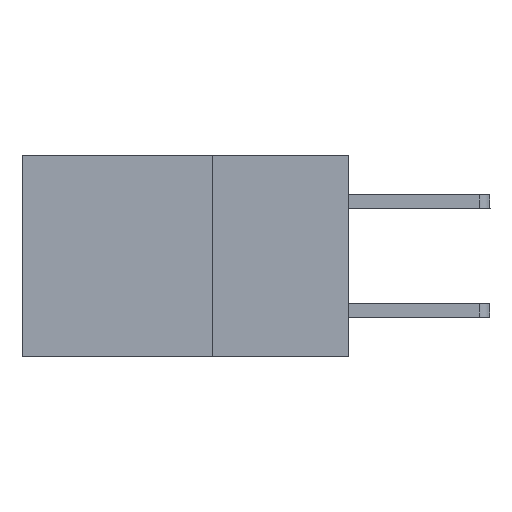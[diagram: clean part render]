
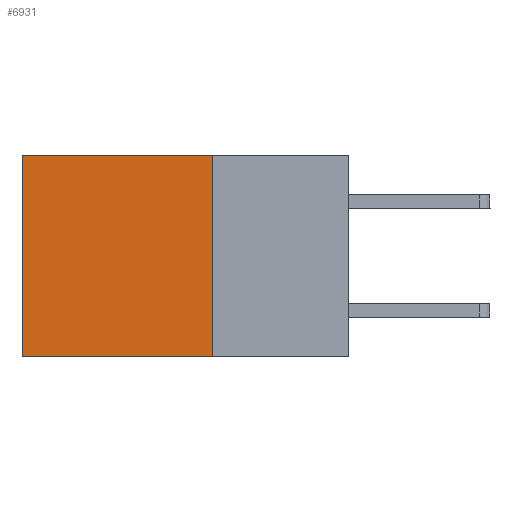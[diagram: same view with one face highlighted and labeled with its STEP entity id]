
A CAD part, left-side view. The second image highlights one B-rep face of the part: STEP entity #6931.
In plain terms, the highlighted planar face has unit normal (-1, 0, 0).
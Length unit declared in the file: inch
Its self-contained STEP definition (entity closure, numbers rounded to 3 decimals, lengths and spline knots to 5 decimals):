
#618 = VERTEX_POINT ( 'NONE', #10238 ) ;
#727 = CARTESIAN_POINT ( 'NONE',  ( 0.298, 0.25, -0.37 ) ) ;
#946 = CARTESIAN_POINT ( 'NONE',  ( 0.298, 0.6, 0. ) ) ;
#1016 = LINE ( 'NONE', #1638, #9282 ) ;
#1069 = ORIENTED_EDGE ( 'NONE', *, *, #3397, .F. ) ;
#1202 = VECTOR ( 'NONE', #9985, 39.37008 ) ;
#1638 = CARTESIAN_POINT ( 'NONE',  ( 0.298, 0.25, 0. ) ) ;
#2792 = DIRECTION ( 'NONE',  ( 0., 0., -1. ) ) ;
#2838 = DIRECTION ( 'NONE',  ( 1., 0., 0. ) ) ;
#3087 = AXIS2_PLACEMENT_3D ( 'NONE', #9989, #2838, #2792 ) ;
#3397 = EDGE_CURVE ( 'NONE', #8082, #6408, #9560, .T. ) ;
#3431 = DIRECTION ( 'NONE',  ( 0., 0., -1. ) ) ;
#3647 = CARTESIAN_POINT ( 'NONE',  ( 0.298, 0.25, 0. ) ) ;
#4001 = ORIENTED_EDGE ( 'NONE', *, *, #9084, .F. ) ;
#4327 = ORIENTED_EDGE ( 'NONE', *, *, #10262, .T. ) ;
#4586 = EDGE_CURVE ( 'NONE', #618, #9806, #6877, .T. ) ;
#5271 = DIRECTION ( 'NONE',  ( 0., 1., 0. ) ) ;
#5978 = CARTESIAN_POINT ( 'NONE',  ( 0.298, 0.6, -0.37 ) ) ;
#6033 = CARTESIAN_POINT ( 'NONE',  ( 0.298, 0.6, 0. ) ) ;
#6408 = VERTEX_POINT ( 'NONE', #5978 ) ;
#6627 = EDGE_LOOP ( 'NONE', ( #4327, #1069, #4001, #9492 ) ) ;
#6817 = CARTESIAN_POINT ( 'NONE',  ( 0.298, 0.25, -0.37 ) ) ;
#6877 = LINE ( 'NONE', #3647, #9443 ) ;
#6931 = ADVANCED_FACE ( 'NONE', ( #9304 ), #9351, .F. ) ;
#8082 = VERTEX_POINT ( 'NONE', #6817 ) ;
#8718 = DIRECTION ( 'NONE',  ( 0., 1., 0. ) ) ;
#9084 = EDGE_CURVE ( 'NONE', #618, #8082, #1016, .T. ) ;
#9147 = LINE ( 'NONE', #946, #1202 ) ;
#9282 = VECTOR ( 'NONE', #3431, 39.37008 ) ;
#9304 = FACE_OUTER_BOUND ( 'NONE', #6627, .T. ) ;
#9351 = PLANE ( 'NONE',  #3087 ) ;
#9443 = VECTOR ( 'NONE', #5271, 39.37008 ) ;
#9492 = ORIENTED_EDGE ( 'NONE', *, *, #4586, .T. ) ;
#9560 = LINE ( 'NONE', #727, #10348 ) ;
#9806 = VERTEX_POINT ( 'NONE', #6033 ) ;
#9985 = DIRECTION ( 'NONE',  ( 0., 0., -1. ) ) ;
#9989 = CARTESIAN_POINT ( 'NONE',  ( 0.298, 0.25, 0. ) ) ;
#10238 = CARTESIAN_POINT ( 'NONE',  ( 0.298, 0.25, 0. ) ) ;
#10262 = EDGE_CURVE ( 'NONE', #9806, #6408, #9147, .T. ) ;
#10348 = VECTOR ( 'NONE', #8718, 39.37008 ) ;
